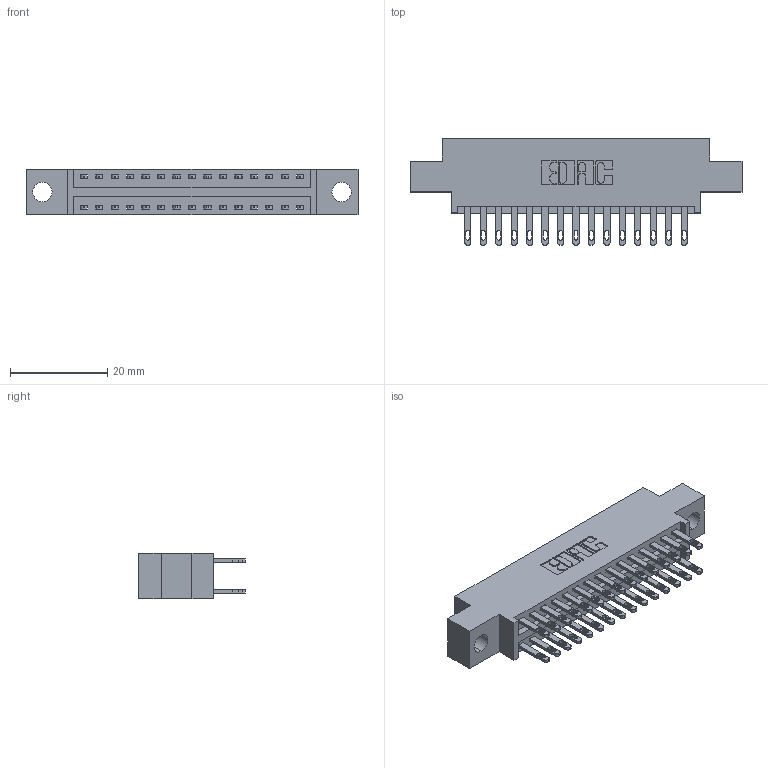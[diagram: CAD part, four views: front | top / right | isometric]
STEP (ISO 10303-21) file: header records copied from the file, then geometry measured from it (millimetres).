
FILE_DESCRIPTION (( 'STEP AP203' ), '1' );
FILE_NAME ('346-030-500-804.STEP', '2022-05-19T15:55:49', ( '' ), ( '' ), 'SwSTEP 2.0', 'SolidWorks 2020', '' );
FILE_SCHEMA (( 'CONFIG_CONTROL_DESIGN' ));
Length unit declared in the file: inch
Products named in the file (3): 345-292-001_345-293-100; 346 Part_0.170 Offset - 0.156 Dia-TH; 346-030-500-804
Assembly tree (31 placements, depth 2):
  346-030-500-804
    346 Part_0.170 Offset - 0.156 Dia-TH
    345-292-001_345-293-100  x30
Bounding box: 68.2 x 21.84 x 9.4 mm (x, y, z)
Volume: 6271.7 mm3; surface area: 8537.9 mm2
Topology: 31 solids, 31 shells, 1580 faces, 4787 edges, 3190 vertices
Faces by surface type: plane 964, cylinder 616
Entity records: 13905 total; most frequent: CARTESIAN_POINT 2334, ORIENTED_EDGE 2266, DIRECTION 2109, EDGE_CURVE 1133, VECTOR 937, LINE 937, VERTEX_POINT 754, AXIS2_PLACEMENT_3D 586
